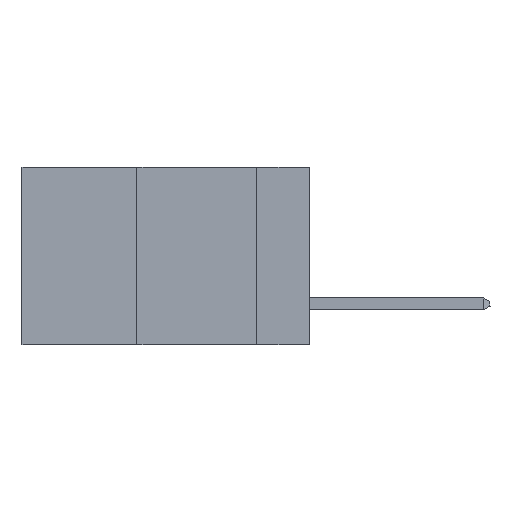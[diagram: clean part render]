
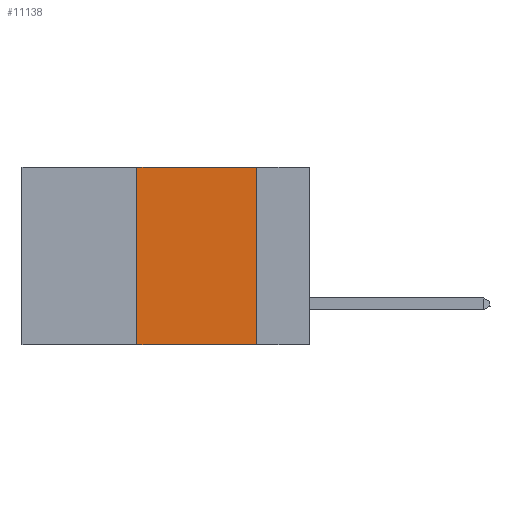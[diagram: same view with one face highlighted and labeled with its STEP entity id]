
A CAD part, left-side view. The second image highlights one B-rep face of the part: STEP entity #11138.
In plain terms, the highlighted planar face has unit normal (-1, 0, 0).
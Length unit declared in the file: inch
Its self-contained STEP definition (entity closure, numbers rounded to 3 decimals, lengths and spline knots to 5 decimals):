
#1278 = ORIENTED_EDGE ( 'NONE', *, *, #15296, .T. ) ;
#1978 = LINE ( 'NONE', #2750, #9762 ) ;
#2134 = LINE ( 'NONE', #14218, #5204 ) ;
#2255 = CARTESIAN_POINT ( 'NONE',  ( 0., 0.11, -0.37 ) ) ;
#2482 = DIRECTION ( 'NONE',  ( 0., 0., 1. ) ) ;
#2750 = CARTESIAN_POINT ( 'NONE',  ( 0., 0.11, 0. ) ) ;
#2753 = DIRECTION ( 'NONE',  ( 1., 0., 0. ) ) ;
#3635 = CARTESIAN_POINT ( 'NONE',  ( 0., 0.6, -0.37 ) ) ;
#3749 = CARTESIAN_POINT ( 'NONE',  ( 0., 0.11, 0. ) ) ;
#3791 = VERTEX_POINT ( 'NONE', #14545 ) ;
#5204 = VECTOR ( 'NONE', #2482, 39.37008 ) ;
#5212 = VECTOR ( 'NONE', #7478, 39.37008 ) ;
#5699 = FACE_OUTER_BOUND ( 'NONE', #12736, .T. ) ;
#6637 = CARTESIAN_POINT ( 'NONE',  ( 0., 0.36, -0.37 ) ) ;
#6789 = CARTESIAN_POINT ( 'NONE',  ( 0., 0.6, 0. ) ) ;
#6900 = DIRECTION ( 'NONE',  ( 0., 0., -1. ) ) ;
#6943 = EDGE_CURVE ( 'NONE', #3791, #7334, #11798, .T. ) ;
#7028 = CARTESIAN_POINT ( 'NONE',  ( 0., 0.6, 0. ) ) ;
#7334 = VERTEX_POINT ( 'NONE', #3749 ) ;
#7379 = EDGE_CURVE ( 'NONE', #11316, #3791, #2134, .T. ) ;
#7478 = DIRECTION ( 'NONE',  ( 0., -1., 0. ) ) ;
#7490 = LINE ( 'NONE', #3635, #5212 ) ;
#8082 = AXIS2_PLACEMENT_3D ( 'NONE', #6789, #2753, #13140 ) ;
#8947 = PLANE ( 'NONE',  #8082 ) ;
#9762 = VECTOR ( 'NONE', #6900, 39.37008 ) ;
#10065 = ORIENTED_EDGE ( 'NONE', *, *, #7379, .F. ) ;
#10299 = VERTEX_POINT ( 'NONE', #2255 ) ;
#11138 = ADVANCED_FACE ( 'NONE', ( #5699 ), #8947, .F. ) ;
#11316 = VERTEX_POINT ( 'NONE', #6637 ) ;
#11798 = LINE ( 'NONE', #7028, #13442 ) ;
#12534 = ORIENTED_EDGE ( 'NONE', *, *, #6943, .F. ) ;
#12736 = EDGE_LOOP ( 'NONE', ( #16516, #12534, #10065, #1278 ) ) ;
#13140 = DIRECTION ( 'NONE',  ( 0., 0., -1. ) ) ;
#13442 = VECTOR ( 'NONE', #15055, 39.37008 ) ;
#13945 = EDGE_CURVE ( 'NONE', #7334, #10299, #1978, .T. ) ;
#14218 = CARTESIAN_POINT ( 'NONE',  ( 0., 0.36, 0. ) ) ;
#14545 = CARTESIAN_POINT ( 'NONE',  ( 0., 0.36, 0. ) ) ;
#15055 = DIRECTION ( 'NONE',  ( 0., -1., 0. ) ) ;
#15296 = EDGE_CURVE ( 'NONE', #11316, #10299, #7490, .T. ) ;
#16516 = ORIENTED_EDGE ( 'NONE', *, *, #13945, .F. ) ;
